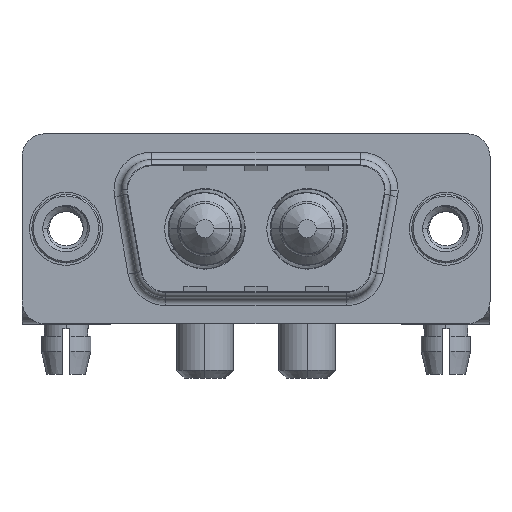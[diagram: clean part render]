
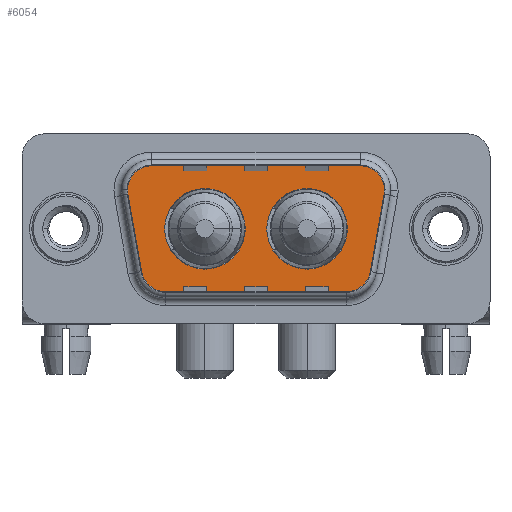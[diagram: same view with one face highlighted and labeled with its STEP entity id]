
A CAD part, top view. The second image highlights one B-rep face of the part: STEP entity #6054.
In plain terms, the highlighted planar face has unit normal (0, 0, 1).
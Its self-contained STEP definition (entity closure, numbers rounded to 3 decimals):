
#144 = CIRCLE ( 'NONE', #11106, 2.65 ) ;
#283 = ORIENTED_EDGE ( 'NONE', *, *, #7059, .T. ) ;
#376 = VERTEX_POINT ( 'NONE', #13249 ) ;
#457 = VERTEX_POINT ( 'NONE', #1876 ) ;
#619 = DIRECTION ( 'NONE',  ( 1., 0., 0. ) ) ;
#786 = CARTESIAN_POINT ( 'NONE',  ( 20.511, -3.247, 0. ) ) ;
#885 = VERTEX_POINT ( 'NONE', #786 ) ;
#908 = CARTESIAN_POINT ( 'NONE',  ( 6.459, -4.9, 0. ) ) ;
#930 = CARTESIAN_POINT ( 'NONE',  ( 6.459, -2.9, 0. ) ) ;
#979 = FACE_OUTER_BOUND ( 'NONE', #1793, .T. ) ;
#1030 = CARTESIAN_POINT ( 'NONE',  ( 21.564, 2.9, 0. ) ) ;
#1078 = ORIENTED_EDGE ( 'NONE', *, *, #10041, .T. ) ;
#1557 = AXIS2_PLACEMENT_3D ( 'NONE', #13740, #10522, #3439 ) ;
#1579 = CIRCLE ( 'NONE', #8887, 2. ) ;
#1793 = EDGE_LOOP ( 'NONE', ( #283, #13704, #12052, #5273, #1078, #11690, #14539, #15026, #13982 ) ) ;
#1876 = CARTESIAN_POINT ( 'NONE',  ( 21.534, 2.553, 0. ) ) ;
#1990 = CARTESIAN_POINT ( 'NONE',  ( 21.534, 2.553, 0. ) ) ;
#2123 = VERTEX_POINT ( 'NONE', #13565 ) ;
#2479 = VERTEX_POINT ( 'NONE', #9575 ) ;
#2741 = AXIS2_PLACEMENT_3D ( 'NONE', #3413, #4792, #6006 ) ;
#3051 = CARTESIAN_POINT ( 'NONE',  ( 5.436, 4.9, 0. ) ) ;
#3132 = EDGE_CURVE ( 'NONE', #885, #457, #12453, .T. ) ;
#3413 = CARTESIAN_POINT ( 'NONE',  ( 5.436, 2.9, 0. ) ) ;
#3429 = DIRECTION ( 'NONE',  ( 0., 0., 1. ) ) ;
#3439 = DIRECTION ( 'NONE',  ( -1., 0., 0. ) ) ;
#3445 = CARTESIAN_POINT ( 'NONE',  ( 19.564, 2.9, 0. ) ) ;
#3518 = DIRECTION ( 'NONE',  ( 0., 0., 1. ) ) ;
#3521 = DIRECTION ( 'NONE',  ( -1., 0., 0. ) ) ;
#3600 = DIRECTION ( 'NONE',  ( 0., 0., 1. ) ) ;
#3686 = VERTEX_POINT ( 'NONE', #1030 ) ;
#3806 = ORIENTED_EDGE ( 'NONE', *, *, #11153, .F. ) ;
#3808 = CIRCLE ( 'NONE', #12337, 2. ) ;
#4351 = FACE_BOUND ( 'NONE', #11176, .T. ) ;
#4504 = CARTESIAN_POINT ( 'NONE',  ( 18.541, -2.9, 0. ) ) ;
#4587 = PLANE ( 'NONE',  #5200 ) ;
#4792 = DIRECTION ( 'NONE',  ( 0., 0., 1. ) ) ;
#4805 = AXIS2_PLACEMENT_3D ( 'NONE', #3445, #3600, #3521 ) ;
#4806 = EDGE_CURVE ( 'NONE', #12408, #376, #6897, .T. ) ;
#4886 = CARTESIAN_POINT ( 'NONE',  ( 3.466, 2.553, 0. ) ) ;
#4918 = DIRECTION ( 'NONE',  ( 0., 0., 1. ) ) ;
#5128 = AXIS2_PLACEMENT_3D ( 'NONE', #9156, #3518, #10448 ) ;
#5200 = AXIS2_PLACEMENT_3D ( 'NONE', #4504, #5569, #9148 ) ;
#5273 = ORIENTED_EDGE ( 'NONE', *, *, #6407, .T. ) ;
#5563 = DIRECTION ( 'NONE',  ( 1., 0., 0. ) ) ;
#5569 = DIRECTION ( 'NONE',  ( 0., 0., 1. ) ) ;
#5596 = DIRECTION ( 'NONE',  ( -1., 0., 0. ) ) ;
#5653 = DIRECTION ( 'NONE',  ( 1., 0., 0. ) ) ;
#6006 = DIRECTION ( 'NONE',  ( 1., 0., 0. ) ) ;
#6054 = ADVANCED_FACE ( 'NONE', ( #8012, #4351, #979 ), #4587, .T. ) ;
#6102 = DIRECTION ( 'NONE',  ( 0.174, -0.985, 0. ) ) ;
#6144 = VERTEX_POINT ( 'NONE', #9376 ) ;
#6201 = ORIENTED_EDGE ( 'NONE', *, *, #11899, .F. ) ;
#6256 = VECTOR ( 'NONE', #9962, 1000. ) ;
#6407 = EDGE_CURVE ( 'NONE', #3686, #6144, #9099, .T. ) ;
#6600 = DIRECTION ( 'NONE',  ( 0.174, 0.985, 0. ) ) ;
#6646 = CARTESIAN_POINT ( 'NONE',  ( 13.21, 0., 0. ) ) ;
#6711 = DIRECTION ( 'NONE',  ( 0., 0., 1. ) ) ;
#6765 = CIRCLE ( 'NONE', #7011, 2.65 ) ;
#6897 = CIRCLE ( 'NONE', #2741, 2. ) ;
#6947 = CARTESIAN_POINT ( 'NONE',  ( 15.86, 0., 0. ) ) ;
#7011 = AXIS2_PLACEMENT_3D ( 'NONE', #6947, #3429, #5563 ) ;
#7059 = EDGE_CURVE ( 'NONE', #2123, #885, #1579, .T. ) ;
#7166 = EDGE_LOOP ( 'NONE', ( #6201, #3806 ) ) ;
#7657 = VERTEX_POINT ( 'NONE', #8428 ) ;
#8012 = FACE_BOUND ( 'NONE', #7166, .T. ) ;
#8015 = VERTEX_POINT ( 'NONE', #9252 ) ;
#8428 = CARTESIAN_POINT ( 'NONE',  ( 18.51, 0., 0. ) ) ;
#8667 = VECTOR ( 'NONE', #6600, 1000. ) ;
#8780 = VECTOR ( 'NONE', #619, 1000. ) ;
#8887 = AXIS2_PLACEMENT_3D ( 'NONE', #10132, #6711, #11339 ) ;
#8977 = EDGE_CURVE ( 'NONE', #2479, #10728, #3808, .T. ) ;
#9099 = CIRCLE ( 'NONE', #1557, 2. ) ;
#9148 = DIRECTION ( 'NONE',  ( 1., 0., 0. ) ) ;
#9156 = CARTESIAN_POINT ( 'NONE',  ( 9.14, 0., 0. ) ) ;
#9252 = CARTESIAN_POINT ( 'NONE',  ( 6.49, 0., 0. ) ) ;
#9376 = CARTESIAN_POINT ( 'NONE',  ( 19.564, 4.9, 0. ) ) ;
#9575 = CARTESIAN_POINT ( 'NONE',  ( 4.489, -3.247, 0. ) ) ;
#9962 = DIRECTION ( 'NONE',  ( -1., 0., 0. ) ) ;
#10041 = EDGE_CURVE ( 'NONE', #6144, #12408, #11308, .T. ) ;
#10132 = CARTESIAN_POINT ( 'NONE',  ( 18.541, -2.9, 0. ) ) ;
#10302 = EDGE_CURVE ( 'NONE', #8015, #10798, #144, .T. ) ;
#10448 = DIRECTION ( 'NONE',  ( 1., 0., 0. ) ) ;
#10521 = ORIENTED_EDGE ( 'NONE', *, *, #10302, .F. ) ;
#10522 = DIRECTION ( 'NONE',  ( 0., 0., 1. ) ) ;
#10713 = EDGE_CURVE ( 'NONE', #457, #3686, #15012, .T. ) ;
#10728 = VERTEX_POINT ( 'NONE', #11757 ) ;
#10758 = CARTESIAN_POINT ( 'NONE',  ( 11.79, 0., 0. ) ) ;
#10798 = VERTEX_POINT ( 'NONE', #10758 ) ;
#11106 = AXIS2_PLACEMENT_3D ( 'NONE', #13145, #4918, #14214 ) ;
#11153 = EDGE_CURVE ( 'NONE', #14743, #7657, #6765, .T. ) ;
#11176 = EDGE_LOOP ( 'NONE', ( #12518, #10521 ) ) ;
#11308 = LINE ( 'NONE', #14903, #6256 ) ;
#11339 = DIRECTION ( 'NONE',  ( 1., 0., 0. ) ) ;
#11450 = DIRECTION ( 'NONE',  ( 0., 0., 1. ) ) ;
#11647 = AXIS2_PLACEMENT_3D ( 'NONE', #13679, #11450, #5653 ) ;
#11690 = ORIENTED_EDGE ( 'NONE', *, *, #4806, .T. ) ;
#11757 = CARTESIAN_POINT ( 'NONE',  ( 6.459, -4.9, 0. ) ) ;
#11899 = EDGE_CURVE ( 'NONE', #7657, #14743, #13602, .T. ) ;
#12052 = ORIENTED_EDGE ( 'NONE', *, *, #10713, .T. ) ;
#12323 = DIRECTION ( 'NONE',  ( 0., 0., 1. ) ) ;
#12337 = AXIS2_PLACEMENT_3D ( 'NONE', #930, #12323, #5596 ) ;
#12408 = VERTEX_POINT ( 'NONE', #3051 ) ;
#12447 = LINE ( 'NONE', #908, #8780 ) ;
#12453 = LINE ( 'NONE', #1990, #8667 ) ;
#12518 = ORIENTED_EDGE ( 'NONE', *, *, #14411, .F. ) ;
#12815 = EDGE_CURVE ( 'NONE', #376, #2479, #12965, .T. ) ;
#12965 = LINE ( 'NONE', #4886, #13856 ) ;
#13145 = CARTESIAN_POINT ( 'NONE',  ( 9.14, 0., 0. ) ) ;
#13249 = CARTESIAN_POINT ( 'NONE',  ( 3.466, 2.553, 0. ) ) ;
#13565 = CARTESIAN_POINT ( 'NONE',  ( 18.541, -4.9, 0. ) ) ;
#13602 = CIRCLE ( 'NONE', #11647, 2.65 ) ;
#13679 = CARTESIAN_POINT ( 'NONE',  ( 15.86, 0., 0. ) ) ;
#13704 = ORIENTED_EDGE ( 'NONE', *, *, #3132, .T. ) ;
#13740 = CARTESIAN_POINT ( 'NONE',  ( 19.564, 2.9, 0. ) ) ;
#13856 = VECTOR ( 'NONE', #6102, 1000. ) ;
#13982 = ORIENTED_EDGE ( 'NONE', *, *, #14239, .T. ) ;
#14214 = DIRECTION ( 'NONE',  ( 1., 0., 0. ) ) ;
#14239 = EDGE_CURVE ( 'NONE', #10728, #2123, #12447, .T. ) ;
#14411 = EDGE_CURVE ( 'NONE', #10798, #8015, #14636, .T. ) ;
#14539 = ORIENTED_EDGE ( 'NONE', *, *, #12815, .T. ) ;
#14636 = CIRCLE ( 'NONE', #5128, 2.65 ) ;
#14743 = VERTEX_POINT ( 'NONE', #6646 ) ;
#14903 = CARTESIAN_POINT ( 'NONE',  ( 5.436, 4.9, 0. ) ) ;
#15012 = CIRCLE ( 'NONE', #4805, 2. ) ;
#15026 = ORIENTED_EDGE ( 'NONE', *, *, #8977, .T. ) ;
